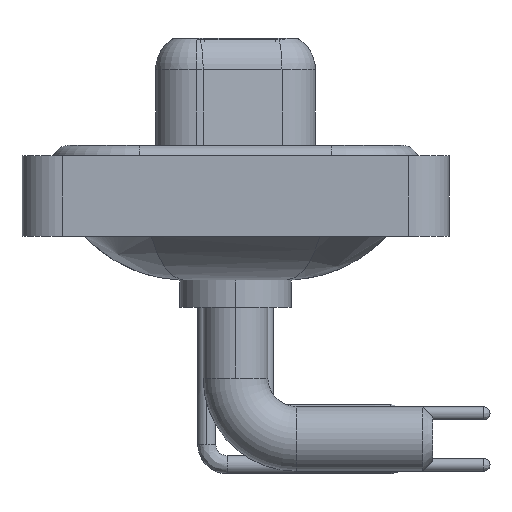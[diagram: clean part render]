
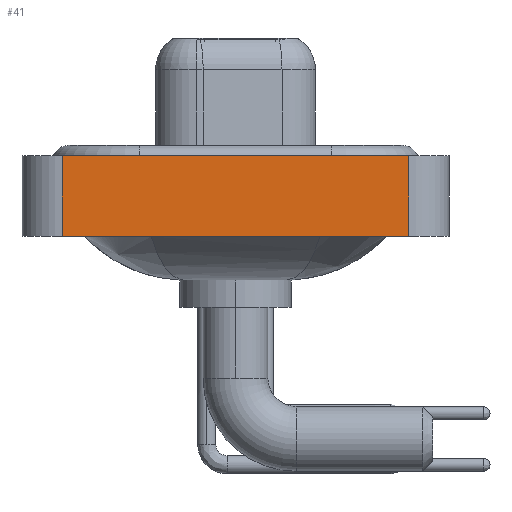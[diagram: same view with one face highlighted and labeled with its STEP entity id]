
A CAD part, left-side view. The second image highlights one B-rep face of the part: STEP entity #41.
In plain terms, the highlighted planar face has unit normal (-1, 0, 0).
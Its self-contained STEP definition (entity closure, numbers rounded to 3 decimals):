
#27 = VECTOR ( 'NONE', #13863, 1000. ) ;
#41 = ADVANCED_FACE ( 'NONE', ( #17060 ), #3042, .T. ) ;
#683 = VECTOR ( 'NONE', #10809, 1000. ) ;
#1172 = VERTEX_POINT ( 'NONE', #20271 ) ;
#2549 = VERTEX_POINT ( 'NONE', #6907 ) ;
#2908 = LINE ( 'NONE', #20055, #683 ) ;
#3042 = PLANE ( 'NONE',  #11411 ) ;
#3044 = EDGE_LOOP ( 'NONE', ( #17828, #13591, #17063, #4366 ) ) ;
#3678 = VECTOR ( 'NONE', #12644, 1000. ) ;
#4366 = ORIENTED_EDGE ( 'NONE', *, *, #11237, .T. ) ;
#4409 = CARTESIAN_POINT ( 'NONE',  ( -7.3, -8.55, 0.4 ) ) ;
#4596 = CARTESIAN_POINT ( 'NONE',  ( -7.3, -8.55, -3.6 ) ) ;
#5810 = CARTESIAN_POINT ( 'NONE',  ( -7.3, -8.55, -3.6 ) ) ;
#6126 = CARTESIAN_POINT ( 'NONE',  ( -7.3, 8.55, 0.4 ) ) ;
#6907 = CARTESIAN_POINT ( 'NONE',  ( -7.3, 8.55, -3.6 ) ) ;
#8098 = CARTESIAN_POINT ( 'NONE',  ( -7.3, -8.55, 0.4 ) ) ;
#8428 = EDGE_CURVE ( 'NONE', #2549, #9161, #2908, .T. ) ;
#9079 = LINE ( 'NONE', #4409, #27 ) ;
#9101 = VERTEX_POINT ( 'NONE', #8098 ) ;
#9161 = VERTEX_POINT ( 'NONE', #6126 ) ;
#9261 = DIRECTION ( 'NONE',  ( 0., 0., 1. ) ) ;
#10730 = VECTOR ( 'NONE', #18775, 1000. ) ;
#10746 = LINE ( 'NONE', #18637, #3678 ) ;
#10809 = DIRECTION ( 'NONE',  ( 0., 0., 1. ) ) ;
#10830 = DIRECTION ( 'NONE',  ( -1., 0., 0. ) ) ;
#11237 = EDGE_CURVE ( 'NONE', #2549, #1172, #10746, .T. ) ;
#11411 = AXIS2_PLACEMENT_3D ( 'NONE', #4596, #10830, #9261 ) ;
#12157 = LINE ( 'NONE', #5810, #10730 ) ;
#12644 = DIRECTION ( 'NONE',  ( 0., -1., 0. ) ) ;
#12665 = EDGE_CURVE ( 'NONE', #9161, #9101, #9079, .T. ) ;
#13591 = ORIENTED_EDGE ( 'NONE', *, *, #12665, .F. ) ;
#13863 = DIRECTION ( 'NONE',  ( 0., -1., 0. ) ) ;
#15168 = EDGE_CURVE ( 'NONE', #1172, #9101, #12157, .T. ) ;
#17060 = FACE_OUTER_BOUND ( 'NONE', #3044, .T. ) ;
#17063 = ORIENTED_EDGE ( 'NONE', *, *, #8428, .F. ) ;
#17828 = ORIENTED_EDGE ( 'NONE', *, *, #15168, .T. ) ;
#18637 = CARTESIAN_POINT ( 'NONE',  ( -7.3, -8.55, -3.6 ) ) ;
#18775 = DIRECTION ( 'NONE',  ( 0., 0., 1. ) ) ;
#20055 = CARTESIAN_POINT ( 'NONE',  ( -7.3, 8.55, -3.6 ) ) ;
#20271 = CARTESIAN_POINT ( 'NONE',  ( -7.3, -8.55, -3.6 ) ) ;
